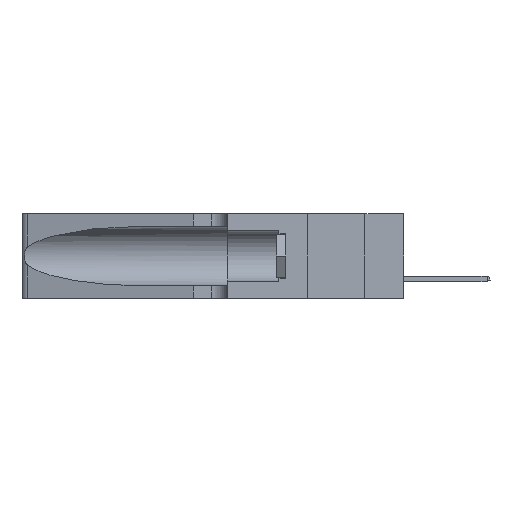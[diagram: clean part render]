
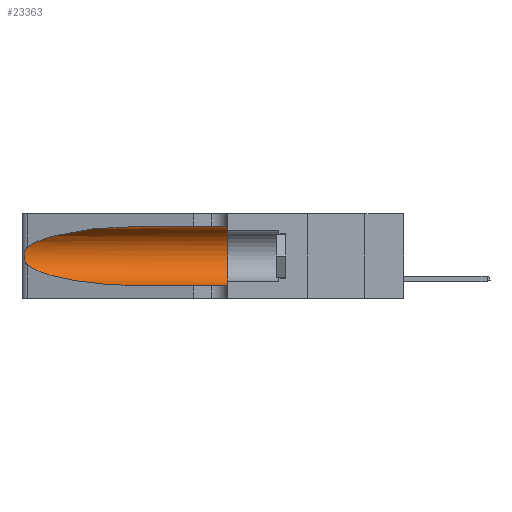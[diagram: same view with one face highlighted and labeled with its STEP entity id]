
A CAD part, left-side view. The second image highlights one B-rep face of the part: STEP entity #23363.
In plain terms, the highlighted cylindrical face has radius 3.308 mm (diameter 6.617 mm), a partial arc.
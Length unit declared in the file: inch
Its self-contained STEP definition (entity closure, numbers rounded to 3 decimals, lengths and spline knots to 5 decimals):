
#168 = CARTESIAN_POINT ( 'NONE',  ( 0.25555, 1.22994, 0.2215 ) ) ;
#201 = CYLINDRICAL_SURFACE ( 'NONE', #17441, 0.13025 ) ;
#302 = ORIENTED_EDGE ( 'NONE', *, *, #15487, .T. ) ;
#793 = EDGE_LOOP ( 'NONE', ( #23812, #24463, #302, #14999, #13171, #23413 ) ) ;
#1461 = CARTESIAN_POINT ( 'NONE',  ( 0.25854, 1.2359, 0.20912 ) ) ;
#2965 = CARTESIAN_POINT ( 'NONE',  ( 0.26017, 1.23833, 0.17102 ) ) ;
#4457 = CARTESIAN_POINT ( 'NONE',  ( 0.26075, 1.23896, 0.19203 ) ) ;
#4468 = CARTESIAN_POINT ( 'NONE',  ( 0.1305, 0.72297, 0.31525 ) ) ;
#4975 = CARTESIAN_POINT ( 'NONE',  ( 0.1305, 1.61858, 0.05475 ) ) ;
#5198 = CARTESIAN_POINT ( 'NONE',  ( 0.25639, 1.23186, 0.15144 ) ) ;
#5264 = VERTEX_POINT ( 'NONE', #18537 ) ;
#7258 = CARTESIAN_POINT ( 'NONE',  ( 0.25487, 1.22718, 0.22369 ) ) ;
#7465 = DIRECTION ( 'NONE',  ( 0., -1., 0. ) ) ;
#9540 = EDGE_CURVE ( 'NONE', #16175, #16959, #18375, .T. ) ;
#9562 = CARTESIAN_POINT ( 'NONE',  ( 0.1305, 1.61858, 0.185 ) ) ;
#9850 = DIRECTION ( 'NONE',  ( 0., 0., 1. ) ) ;
#10143 = LINE ( 'NONE', #12990, #20503 ) ;
#10678 = CARTESIAN_POINT ( 'NONE',  ( 0.25487, 1.22718, 0.14631 ) ) ;
#10865 = CARTESIAN_POINT ( 'NONE',  ( 0.1305, 0.72297, 0.05475 ) ) ;
#11051 = VERTEX_POINT ( 'NONE', #21365 ) ;
#11938 =( BOUNDED_CURVE ( )  B_SPLINE_CURVE ( 3, ( #17953, #20537, #27324, #24810 ),
 .UNSPECIFIED., .F., .F. ) 
 B_SPLINE_CURVE_WITH_KNOTS ( ( 4, 4 ),
 ( 1.5708, 2.84003 ),
 .UNSPECIFIED. ) 
 CURVE ( )  GEOMETRIC_REPRESENTATION_ITEM ( )  RATIONAL_B_SPLINE_CURVE ( ( 1., 0.87, 0.87, 1. ) ) 
 REPRESENTATION_ITEM ( '' )  );
#12136 = CARTESIAN_POINT ( 'NONE',  ( 0.1305, 0.35, 0.185 ) ) ;
#12990 = CARTESIAN_POINT ( 'NONE',  ( 0.1305, 1.61858, 0.31525 ) ) ;
#13171 = ORIENTED_EDGE ( 'NONE', *, *, #27106, .F. ) ;
#13459 = CARTESIAN_POINT ( 'NONE',  ( 0.25856, 1.23593, 0.16098 ) ) ;
#13841 = CARTESIAN_POINT ( 'NONE',  ( 0.25639, 1.23184, 0.21858 ) ) ;
#14999 = ORIENTED_EDGE ( 'NONE', *, *, #24612, .T. ) ;
#15322 = CARTESIAN_POINT ( 'NONE',  ( 0.25487, 1.22718, 0.22369 ) ) ;
#15487 = EDGE_CURVE ( 'NONE', #16959, #23851, #23828, .T. ) ;
#16072 = VECTOR ( 'NONE', #7465, 39.37008 ) ;
#16175 = VERTEX_POINT ( 'NONE', #7258 ) ;
#16784 = CARTESIAN_POINT ( 'NONE',  ( 0.25789, 1.23486, 0.15765 ) ) ;
#16959 = VERTEX_POINT ( 'NONE', #17201 ) ;
#16962 = DIRECTION ( 'NONE',  ( 0., 1., 0. ) ) ;
#17201 = CARTESIAN_POINT ( 'NONE',  ( 0.25487, 1.22718, 0.14631 ) ) ;
#17441 = AXIS2_PLACEMENT_3D ( 'NONE', #9562, #27943, #23221 ) ;
#17953 = CARTESIAN_POINT ( 'NONE',  ( 0.1305, 0.72297, 0.31525 ) ) ;
#18375 = B_SPLINE_CURVE_WITH_KNOTS ( 'NONE', 3,
 ( #15322, #168, #13841, #22245, #1461, #27401, #4457, #27997, #2965, #13459, #16784, #5198, #28357, #18875 ),
 .UNSPECIFIED., .F., .F.,
 ( 4, 2, 2, 2, 2, 2, 4 ),
 ( 0., 0.00027, 0.00053, 0.00107, 0.0016, 0.00187, 0.00214 ),
 .UNSPECIFIED. ) ;
#18537 = CARTESIAN_POINT ( 'NONE',  ( 0.1305, 0.35, 0.05475 ) ) ;
#18875 = CARTESIAN_POINT ( 'NONE',  ( 0.25487, 1.22718, 0.14631 ) ) ;
#20503 = VECTOR ( 'NONE', #22065, 39.37008 ) ;
#20537 = CARTESIAN_POINT ( 'NONE',  ( 0.18966, 0.96281, 0.31525 ) ) ;
#21048 = CIRCLE ( 'NONE', #25605, 0.13025 ) ;
#21365 = CARTESIAN_POINT ( 'NONE',  ( 0.1305, 0.35, 0.31525 ) ) ;
#22031 = VERTEX_POINT ( 'NONE', #4468 ) ;
#22065 = DIRECTION ( 'NONE',  ( 0., -1., 0. ) ) ;
#22245 = CARTESIAN_POINT ( 'NONE',  ( 0.25787, 1.23484, 0.2124 ) ) ;
#22453 = EDGE_CURVE ( 'NONE', #22031, #11051, #10143, .T. ) ;
#23221 = DIRECTION ( 'NONE',  ( 0., 0., -1. ) ) ;
#23363 = ADVANCED_FACE ( 'NONE', ( #26598 ), #201, .F. ) ;
#23413 = ORIENTED_EDGE ( 'NONE', *, *, #22453, .F. ) ;
#23812 = ORIENTED_EDGE ( 'NONE', *, *, #24489, .T. ) ;
#23828 =( BOUNDED_CURVE ( )  B_SPLINE_CURVE ( 3, ( #10678, #24850, #27156, #24952 ),
 .UNSPECIFIED., .F., .F. ) 
 B_SPLINE_CURVE_WITH_KNOTS ( ( 4, 4 ),
 ( 3.44316, 4.71239 ),
 .UNSPECIFIED. ) 
 CURVE ( )  GEOMETRIC_REPRESENTATION_ITEM ( )  RATIONAL_B_SPLINE_CURVE ( ( 1., 0.87, 0.87, 1. ) ) 
 REPRESENTATION_ITEM ( '' )  );
#23851 = VERTEX_POINT ( 'NONE', #10865 ) ;
#24463 = ORIENTED_EDGE ( 'NONE', *, *, #9540, .T. ) ;
#24489 = EDGE_CURVE ( 'NONE', #22031, #16175, #11938, .T. ) ;
#24612 = EDGE_CURVE ( 'NONE', #23851, #5264, #26073, .T. ) ;
#24810 = CARTESIAN_POINT ( 'NONE',  ( 0.25487, 1.22718, 0.22369 ) ) ;
#24850 = CARTESIAN_POINT ( 'NONE',  ( 0.2373, 1.15595, 0.08982 ) ) ;
#24952 = CARTESIAN_POINT ( 'NONE',  ( 0.1305, 0.72297, 0.05475 ) ) ;
#25605 = AXIS2_PLACEMENT_3D ( 'NONE', #12136, #16962, #9850 ) ;
#26073 = LINE ( 'NONE', #4975, #16072 ) ;
#26598 = FACE_OUTER_BOUND ( 'NONE', #793, .T. ) ;
#27106 = EDGE_CURVE ( 'NONE', #11051, #5264, #21048, .T. ) ;
#27156 = CARTESIAN_POINT ( 'NONE',  ( 0.18966, 0.96281, 0.05475 ) ) ;
#27324 = CARTESIAN_POINT ( 'NONE',  ( 0.2373, 1.15595, 0.28018 ) ) ;
#27401 = CARTESIAN_POINT ( 'NONE',  ( 0.26018, 1.23835, 0.19895 ) ) ;
#27943 = DIRECTION ( 'NONE',  ( 0., -1., 0. ) ) ;
#27997 = CARTESIAN_POINT ( 'NONE',  ( 0.26075, 1.23896, 0.178 ) ) ;
#28357 = CARTESIAN_POINT ( 'NONE',  ( 0.25555, 1.22993, 0.14849 ) ) ;
